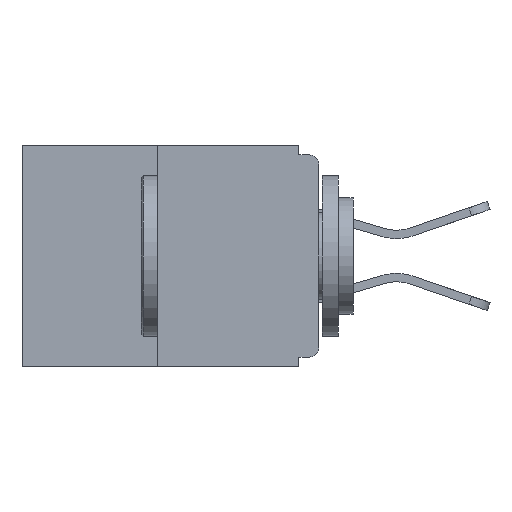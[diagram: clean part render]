
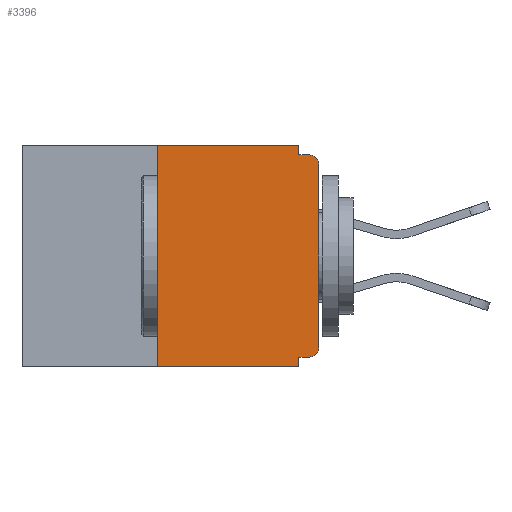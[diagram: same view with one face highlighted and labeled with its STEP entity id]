
A CAD part, left-side view. The second image highlights one B-rep face of the part: STEP entity #3396.
In plain terms, the highlighted planar face has unit normal (-1, 0, 0).
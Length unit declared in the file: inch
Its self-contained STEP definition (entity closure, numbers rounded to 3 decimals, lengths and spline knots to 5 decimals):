
#43 = EDGE_CURVE ( 'NONE', #9830, #1957, #4284, .T. ) ;
#198 = DIRECTION ( 'NONE',  ( 0., -1., 0. ) ) ;
#272 = CARTESIAN_POINT ( 'NONE',  ( 0., 0.031, 0. ) ) ;
#443 = VERTEX_POINT ( 'NONE', #6541 ) ;
#819 = EDGE_CURVE ( 'NONE', #7506, #3256, #12078, .T. ) ;
#906 = LINE ( 'NONE', #12152, #3177 ) ;
#1064 = CARTESIAN_POINT ( 'NONE',  ( 0., 0., -0.015 ) ) ;
#1444 = DIRECTION ( 'NONE',  ( 0., 0., -1. ) ) ;
#1645 = VECTOR ( 'NONE', #198, 39.37008 ) ;
#1957 = VERTEX_POINT ( 'NONE', #14475 ) ;
#2081 = EDGE_CURVE ( 'NONE', #11634, #443, #10315, .T. ) ;
#2189 = DIRECTION ( 'NONE',  ( 1., 0., 0. ) ) ;
#2510 = CARTESIAN_POINT ( 'NONE',  ( 0., 0.46, -0.343 ) ) ;
#2711 = FACE_OUTER_BOUND ( 'NONE', #7724, .T. ) ;
#2938 = VECTOR ( 'NONE', #12309, 39.37008 ) ;
#2944 = CARTESIAN_POINT ( 'NONE',  ( 0., 0.031, -0.343 ) ) ;
#2967 = VERTEX_POINT ( 'NONE', #6446 ) ;
#3101 = CARTESIAN_POINT ( 'NONE',  ( 0., 0.015, -0.328 ) ) ;
#3177 = VECTOR ( 'NONE', #14457, 39.37008 ) ;
#3256 = VERTEX_POINT ( 'NONE', #11131 ) ;
#3319 = ORIENTED_EDGE ( 'NONE', *, *, #13422, .T. ) ;
#3396 = ADVANCED_FACE ( 'NONE', ( #2711 ), #11328, .F. ) ;
#3577 = ORIENTED_EDGE ( 'NONE', *, *, #8265, .T. ) ;
#4121 = AXIS2_PLACEMENT_3D ( 'NONE', #9334, #4703, #1444 ) ;
#4284 = LINE ( 'NONE', #5348, #11851 ) ;
#4342 = ORIENTED_EDGE ( 'NONE', *, *, #43, .F. ) ;
#4425 = DIRECTION ( 'NONE',  ( 0., 0., -1. ) ) ;
#4672 = DIRECTION ( 'NONE',  ( -1., 0., 0. ) ) ;
#4696 = CIRCLE ( 'NONE', #6731, 0.015 ) ;
#4703 = DIRECTION ( 'NONE',  ( -1., 0., 0. ) ) ;
#4705 = EDGE_CURVE ( 'NONE', #1957, #5223, #6883, .T. ) ;
#4876 = EDGE_CURVE ( 'NONE', #3256, #2967, #7386, .T. ) ;
#5223 = VERTEX_POINT ( 'NONE', #13925 ) ;
#5348 = CARTESIAN_POINT ( 'NONE',  ( 0., 0.031, 0. ) ) ;
#5609 = ORIENTED_EDGE ( 'NONE', *, *, #13991, .T. ) ;
#5635 = ORIENTED_EDGE ( 'NONE', *, *, #4876, .F. ) ;
#5813 = DIRECTION ( 'NONE',  ( 0., 0., 1. ) ) ;
#5947 = CARTESIAN_POINT ( 'NONE',  ( 0., 0.015, -0.313 ) ) ;
#6044 = AXIS2_PLACEMENT_3D ( 'NONE', #14455, #2189, #4425 ) ;
#6284 = DIRECTION ( 'NONE',  ( 0., 0., -1. ) ) ;
#6446 = CARTESIAN_POINT ( 'NONE',  ( 0., 0.031, -0.343 ) ) ;
#6502 = EDGE_CURVE ( 'NONE', #7506, #8840, #4696, .T. ) ;
#6541 = CARTESIAN_POINT ( 'NONE',  ( 0., 0.25, 0. ) ) ;
#6660 = ORIENTED_EDGE ( 'NONE', *, *, #6502, .T. ) ;
#6731 = AXIS2_PLACEMENT_3D ( 'NONE', #5947, #4672, #13687 ) ;
#6883 = LINE ( 'NONE', #1064, #11974 ) ;
#7121 = VECTOR ( 'NONE', #5813, 39.37008 ) ;
#7134 = LINE ( 'NONE', #14339, #2938 ) ;
#7386 = LINE ( 'NONE', #2944, #9167 ) ;
#7506 = VERTEX_POINT ( 'NONE', #3101 ) ;
#7724 = EDGE_LOOP ( 'NONE', ( #14347, #13407, #5609, #5635, #9052, #6660, #3577, #3319, #13964, #4342 ) ) ;
#8113 = CARTESIAN_POINT ( 'NONE',  ( 0., 0., -0.03 ) ) ;
#8265 = EDGE_CURVE ( 'NONE', #8840, #10797, #7134, .T. ) ;
#8402 = CARTESIAN_POINT ( 'NONE',  ( 0., 0., -0.313 ) ) ;
#8477 = CIRCLE ( 'NONE', #4121, 0.015 ) ;
#8840 = VERTEX_POINT ( 'NONE', #8402 ) ;
#8885 = DIRECTION ( 'NONE',  ( 0., -1., 0. ) ) ;
#9052 = ORIENTED_EDGE ( 'NONE', *, *, #819, .F. ) ;
#9079 = VECTOR ( 'NONE', #12830, 39.37008 ) ;
#9167 = VECTOR ( 'NONE', #6284, 39.37008 ) ;
#9334 = CARTESIAN_POINT ( 'NONE',  ( 0., 0.015, -0.03 ) ) ;
#9830 = VERTEX_POINT ( 'NONE', #272 ) ;
#10315 = LINE ( 'NONE', #12479, #7121 ) ;
#10797 = VERTEX_POINT ( 'NONE', #8113 ) ;
#11131 = CARTESIAN_POINT ( 'NONE',  ( 0., 0.031, -0.328 ) ) ;
#11230 = DIRECTION ( 'NONE',  ( 0., 0., -1. ) ) ;
#11328 = PLANE ( 'NONE',  #6044 ) ;
#11633 = CARTESIAN_POINT ( 'NONE',  ( 0., 0., -0.328 ) ) ;
#11634 = VERTEX_POINT ( 'NONE', #14267 ) ;
#11689 = EDGE_CURVE ( 'NONE', #443, #9830, #906, .T. ) ;
#11851 = VECTOR ( 'NONE', #11230, 39.37008 ) ;
#11974 = VECTOR ( 'NONE', #8885, 39.37008 ) ;
#12078 = LINE ( 'NONE', #11633, #9079 ) ;
#12152 = CARTESIAN_POINT ( 'NONE',  ( 0., 0.46, 0. ) ) ;
#12309 = DIRECTION ( 'NONE',  ( 0., 0., 1. ) ) ;
#12479 = CARTESIAN_POINT ( 'NONE',  ( 0., 0.25, 0. ) ) ;
#12830 = DIRECTION ( 'NONE',  ( 0., 1., 0. ) ) ;
#13407 = ORIENTED_EDGE ( 'NONE', *, *, #2081, .F. ) ;
#13422 = EDGE_CURVE ( 'NONE', #10797, #5223, #8477, .T. ) ;
#13687 = DIRECTION ( 'NONE',  ( 0., 0., -1. ) ) ;
#13891 = LINE ( 'NONE', #2510, #1645 ) ;
#13925 = CARTESIAN_POINT ( 'NONE',  ( 0., 0.015, -0.015 ) ) ;
#13964 = ORIENTED_EDGE ( 'NONE', *, *, #4705, .F. ) ;
#13991 = EDGE_CURVE ( 'NONE', #11634, #2967, #13891, .T. ) ;
#14267 = CARTESIAN_POINT ( 'NONE',  ( 0., 0.25, -0.343 ) ) ;
#14339 = CARTESIAN_POINT ( 'NONE',  ( 0., 0., 0. ) ) ;
#14347 = ORIENTED_EDGE ( 'NONE', *, *, #11689, .F. ) ;
#14455 = CARTESIAN_POINT ( 'NONE',  ( 0., 0.46, 0. ) ) ;
#14457 = DIRECTION ( 'NONE',  ( 0., -1., 0. ) ) ;
#14475 = CARTESIAN_POINT ( 'NONE',  ( 0., 0.031, -0.015 ) ) ;
